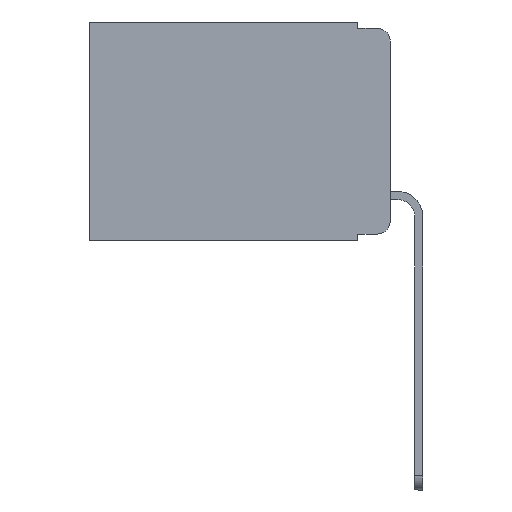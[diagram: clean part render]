
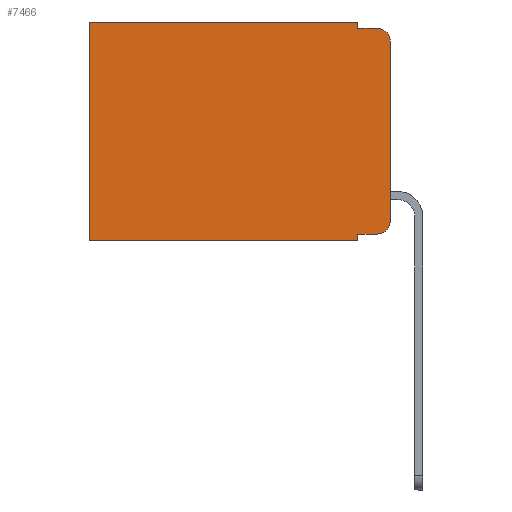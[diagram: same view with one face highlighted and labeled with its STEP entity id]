
A CAD part, left-side view. The second image highlights one B-rep face of the part: STEP entity #7466.
In plain terms, the highlighted planar face has unit normal (-1, 0, 0).
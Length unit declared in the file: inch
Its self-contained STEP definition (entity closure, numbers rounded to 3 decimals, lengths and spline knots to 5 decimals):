
#414 = CARTESIAN_POINT ( 'NONE',  ( 0.298, 0.051, -0.01 ) ) ;
#529 = VERTEX_POINT ( 'NONE', #14434 ) ;
#745 = DIRECTION ( 'NONE',  ( 0., -1., 0. ) ) ;
#923 = LINE ( 'NONE', #2542, #6875 ) ;
#1115 = VERTEX_POINT ( 'NONE', #9152 ) ;
#1486 = LINE ( 'NONE', #17177, #4343 ) ;
#1497 = VERTEX_POINT ( 'NONE', #1922 ) ;
#1901 = DIRECTION ( 'NONE',  ( 0., 0., -1. ) ) ;
#1913 = DIRECTION ( 'NONE',  ( 1., 0., 0. ) ) ;
#1922 = CARTESIAN_POINT ( 'NONE',  ( 0.298, 0.02, -0.333 ) ) ;
#2542 = CARTESIAN_POINT ( 'NONE',  ( 0.298, 0., 0. ) ) ;
#2708 = ORIENTED_EDGE ( 'NONE', *, *, #19057, .T. ) ;
#2767 = EDGE_CURVE ( 'NONE', #17301, #18011, #6652, .T. ) ;
#3377 = DIRECTION ( 'NONE',  ( -1., 0., 0. ) ) ;
#3567 = ORIENTED_EDGE ( 'NONE', *, *, #21756, .T. ) ;
#3895 = ORIENTED_EDGE ( 'NONE', *, *, #15975, .F. ) ;
#4343 = VECTOR ( 'NONE', #13958, 39.37008 ) ;
#4377 = DIRECTION ( 'NONE',  ( 0., 1., 0. ) ) ;
#5027 = CARTESIAN_POINT ( 'NONE',  ( 0.298, 0., 0. ) ) ;
#5670 = EDGE_CURVE ( 'NONE', #529, #20451, #6199, .T. ) ;
#6199 = LINE ( 'NONE', #16290, #12782 ) ;
#6259 = VERTEX_POINT ( 'NONE', #8670 ) ;
#6652 = LINE ( 'NONE', #11925, #15864 ) ;
#6875 = VECTOR ( 'NONE', #4377, 39.37008 ) ;
#7030 = CARTESIAN_POINT ( 'NONE',  ( 0.298, 0.051, -0.01 ) ) ;
#7132 = CARTESIAN_POINT ( 'NONE',  ( 0.298, 0.473, -0.343 ) ) ;
#7243 = CARTESIAN_POINT ( 'NONE',  ( 0.298, 0.051, -0.333 ) ) ;
#7402 = LINE ( 'NONE', #414, #11006 ) ;
#7423 = CARTESIAN_POINT ( 'NONE',  ( 0.298, 0.473, 0. ) ) ;
#7466 = ADVANCED_FACE ( 'NONE', ( #13820 ), #13935, .F. ) ;
#7534 = ORIENTED_EDGE ( 'NONE', *, *, #22348, .T. ) ;
#7756 = CARTESIAN_POINT ( 'NONE',  ( 0.298, 0.051, 0. ) ) ;
#7906 = VECTOR ( 'NONE', #1901, 39.37008 ) ;
#7971 = ORIENTED_EDGE ( 'NONE', *, *, #10837, .T. ) ;
#8670 = CARTESIAN_POINT ( 'NONE',  ( 0.298, 0., -0.313 ) ) ;
#8924 = EDGE_CURVE ( 'NONE', #18011, #16961, #7402, .T. ) ;
#8988 = ORIENTED_EDGE ( 'NONE', *, *, #19813, .F. ) ;
#9152 = CARTESIAN_POINT ( 'NONE',  ( 0.298, 0.473, 0. ) ) ;
#9458 = CARTESIAN_POINT ( 'NONE',  ( 0.298, 0., 0. ) ) ;
#10256 = AXIS2_PLACEMENT_3D ( 'NONE', #5027, #1913, #20816 ) ;
#10837 = EDGE_CURVE ( 'NONE', #20577, #16961, #12899, .T. ) ;
#11006 = VECTOR ( 'NONE', #745, 39.37008 ) ;
#11474 = CARTESIAN_POINT ( 'NONE',  ( 0.298, 0.02, -0.03 ) ) ;
#11540 = CIRCLE ( 'NONE', #15190, 0.02 ) ;
#11925 = CARTESIAN_POINT ( 'NONE',  ( 0.298, 0.051, 0. ) ) ;
#11939 = VERTEX_POINT ( 'NONE', #7243 ) ;
#12782 = VECTOR ( 'NONE', #20181, 39.37008 ) ;
#12899 = CIRCLE ( 'NONE', #21678, 0.02 ) ;
#13167 = CARTESIAN_POINT ( 'NONE',  ( 0.298, 0., -0.03 ) ) ;
#13402 = CARTESIAN_POINT ( 'NONE',  ( 0.298, 0.02, -0.01 ) ) ;
#13575 = ORIENTED_EDGE ( 'NONE', *, *, #5670, .F. ) ;
#13820 = FACE_OUTER_BOUND ( 'NONE', #20509, .T. ) ;
#13935 = PLANE ( 'NONE',  #10256 ) ;
#13958 = DIRECTION ( 'NONE',  ( 0., -1., 0. ) ) ;
#14080 = EDGE_CURVE ( 'NONE', #1115, #20451, #17846, .T. ) ;
#14395 = DIRECTION ( 'NONE',  ( 0., 0., -1. ) ) ;
#14407 = ORIENTED_EDGE ( 'NONE', *, *, #8924, .F. ) ;
#14434 = CARTESIAN_POINT ( 'NONE',  ( 0.298, 0.051, -0.343 ) ) ;
#14725 = LINE ( 'NONE', #9458, #18442 ) ;
#15025 = DIRECTION ( 'NONE',  ( 0., 0., -1. ) ) ;
#15190 = AXIS2_PLACEMENT_3D ( 'NONE', #15385, #3377, #18826 ) ;
#15385 = CARTESIAN_POINT ( 'NONE',  ( 0.298, 0.02, -0.313 ) ) ;
#15864 = VECTOR ( 'NONE', #19136, 39.37008 ) ;
#15975 = EDGE_CURVE ( 'NONE', #20577, #6259, #14725, .T. ) ;
#16248 = ORIENTED_EDGE ( 'NONE', *, *, #14080, .T. ) ;
#16290 = CARTESIAN_POINT ( 'NONE',  ( 0.298, 0., -0.343 ) ) ;
#16462 = DIRECTION ( 'NONE',  ( 0., 0., -1. ) ) ;
#16961 = VERTEX_POINT ( 'NONE', #13402 ) ;
#17177 = CARTESIAN_POINT ( 'NONE',  ( 0.298, 0.051, -0.333 ) ) ;
#17301 = VERTEX_POINT ( 'NONE', #7756 ) ;
#17846 = LINE ( 'NONE', #7423, #18085 ) ;
#18011 = VERTEX_POINT ( 'NONE', #7030 ) ;
#18085 = VECTOR ( 'NONE', #14395, 39.37008 ) ;
#18442 = VECTOR ( 'NONE', #16462, 39.37008 ) ;
#18472 = DIRECTION ( 'NONE',  ( -1., 0., 0. ) ) ;
#18634 = ORIENTED_EDGE ( 'NONE', *, *, #2767, .F. ) ;
#18826 = DIRECTION ( 'NONE',  ( 0., 0., -1. ) ) ;
#18976 = LINE ( 'NONE', #20926, #7906 ) ;
#19057 = EDGE_CURVE ( 'NONE', #1497, #6259, #11540, .T. ) ;
#19136 = DIRECTION ( 'NONE',  ( 0., 0., -1. ) ) ;
#19813 = EDGE_CURVE ( 'NONE', #11939, #529, #18976, .T. ) ;
#20181 = DIRECTION ( 'NONE',  ( 0., 1., 0. ) ) ;
#20451 = VERTEX_POINT ( 'NONE', #7132 ) ;
#20509 = EDGE_LOOP ( 'NONE', ( #3895, #7971, #14407, #18634, #3567, #16248, #13575, #8988, #7534, #2708 ) ) ;
#20577 = VERTEX_POINT ( 'NONE', #13167 ) ;
#20816 = DIRECTION ( 'NONE',  ( 0., 0., -1. ) ) ;
#20926 = CARTESIAN_POINT ( 'NONE',  ( 0.298, 0.051, 0. ) ) ;
#21678 = AXIS2_PLACEMENT_3D ( 'NONE', #11474, #18472, #15025 ) ;
#21756 = EDGE_CURVE ( 'NONE', #17301, #1115, #923, .T. ) ;
#22348 = EDGE_CURVE ( 'NONE', #11939, #1497, #1486, .T. ) ;
